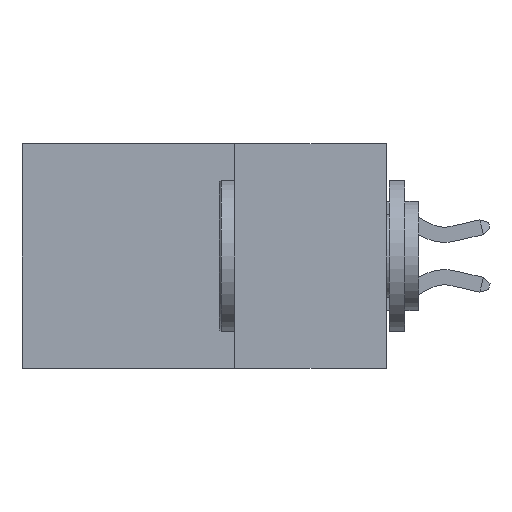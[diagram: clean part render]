
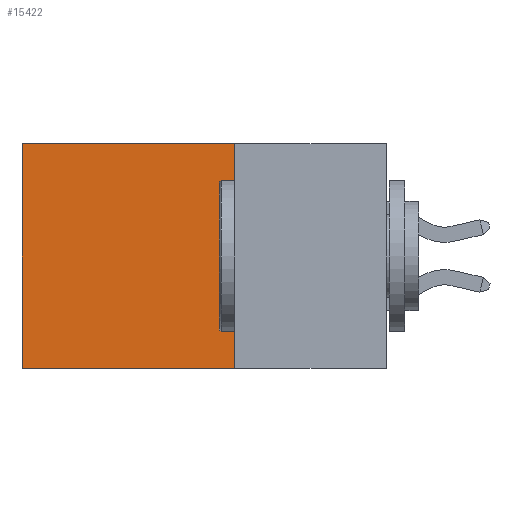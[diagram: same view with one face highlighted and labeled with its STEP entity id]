
A CAD part, left-side view. The second image highlights one B-rep face of the part: STEP entity #15422.
In plain terms, the highlighted planar face has unit normal (-1, 0, 0).
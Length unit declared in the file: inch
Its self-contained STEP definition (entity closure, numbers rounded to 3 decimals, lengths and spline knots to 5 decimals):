
#981 = VERTEX_POINT ( 'NONE', #5815 ) ;
#1479 = EDGE_CURVE ( 'NONE', #981, #2285, #13122, .T. ) ;
#1716 = VECTOR ( 'NONE', #13775, 39.37008 ) ;
#1751 = VERTEX_POINT ( 'NONE', #7414 ) ;
#1793 = EDGE_CURVE ( 'NONE', #1751, #6521, #5164, .T. ) ;
#1883 = CARTESIAN_POINT ( 'NONE',  ( 0.2615, 0.25, -0.37 ) ) ;
#2285 = VERTEX_POINT ( 'NONE', #11274 ) ;
#3115 = FACE_OUTER_BOUND ( 'NONE', #4909, .T. ) ;
#4909 = EDGE_LOOP ( 'NONE', ( #12948, #16542, #14726, #8181 ) ) ;
#5164 = LINE ( 'NONE', #6210, #9130 ) ;
#5296 = LINE ( 'NONE', #13873, #1716 ) ;
#5747 = DIRECTION ( 'NONE',  ( 0., 1., 0. ) ) ;
#5782 = AXIS2_PLACEMENT_3D ( 'NONE', #14407, #6798, #15592 ) ;
#5815 = CARTESIAN_POINT ( 'NONE',  ( 0.2615, 0.25, -0.37 ) ) ;
#6210 = CARTESIAN_POINT ( 'NONE',  ( 0.2615, 0.25, 0. ) ) ;
#6286 = CARTESIAN_POINT ( 'NONE',  ( 0.2615, 0.6, 0. ) ) ;
#6521 = VERTEX_POINT ( 'NONE', #6286 ) ;
#6798 = DIRECTION ( 'NONE',  ( 1., 0., 0. ) ) ;
#7414 = CARTESIAN_POINT ( 'NONE',  ( 0.2615, 0.25, 0. ) ) ;
#7817 = EDGE_CURVE ( 'NONE', #1751, #981, #15831, .T. ) ;
#7834 = DIRECTION ( 'NONE',  ( 0., 1., 0. ) ) ;
#8087 = PLANE ( 'NONE',  #5782 ) ;
#8181 = ORIENTED_EDGE ( 'NONE', *, *, #1793, .T. ) ;
#9130 = VECTOR ( 'NONE', #5747, 39.37008 ) ;
#9739 = VECTOR ( 'NONE', #7834, 39.37008 ) ;
#11274 = CARTESIAN_POINT ( 'NONE',  ( 0.2615, 0.6, -0.37 ) ) ;
#11364 = CARTESIAN_POINT ( 'NONE',  ( 0.2615, 0.25, -0.37 ) ) ;
#11482 = DIRECTION ( 'NONE',  ( 0., 0., -1. ) ) ;
#12104 = EDGE_CURVE ( 'NONE', #6521, #2285, #5296, .T. ) ;
#12681 = VECTOR ( 'NONE', #11482, 39.37008 ) ;
#12948 = ORIENTED_EDGE ( 'NONE', *, *, #12104, .T. ) ;
#13122 = LINE ( 'NONE', #1883, #9739 ) ;
#13775 = DIRECTION ( 'NONE',  ( 0., 0., -1. ) ) ;
#13873 = CARTESIAN_POINT ( 'NONE',  ( 0.2615, 0.6, -0.37 ) ) ;
#14407 = CARTESIAN_POINT ( 'NONE',  ( 0.2615, 0.25, -0.37 ) ) ;
#14726 = ORIENTED_EDGE ( 'NONE', *, *, #7817, .F. ) ;
#15422 = ADVANCED_FACE ( 'NONE', ( #3115 ), #8087, .F. ) ;
#15592 = DIRECTION ( 'NONE',  ( 0., 0., -1. ) ) ;
#15831 = LINE ( 'NONE', #11364, #12681 ) ;
#16542 = ORIENTED_EDGE ( 'NONE', *, *, #1479, .F. ) ;
